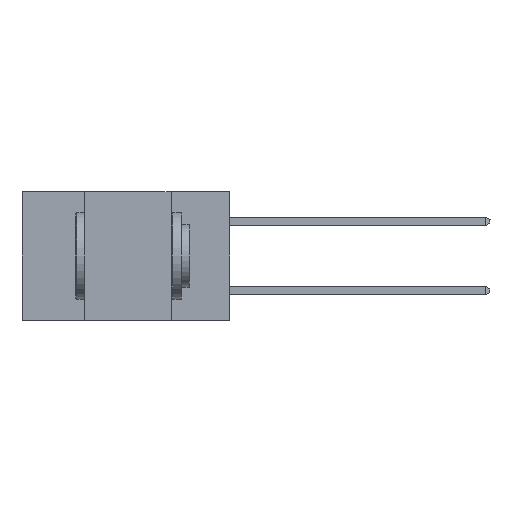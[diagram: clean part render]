
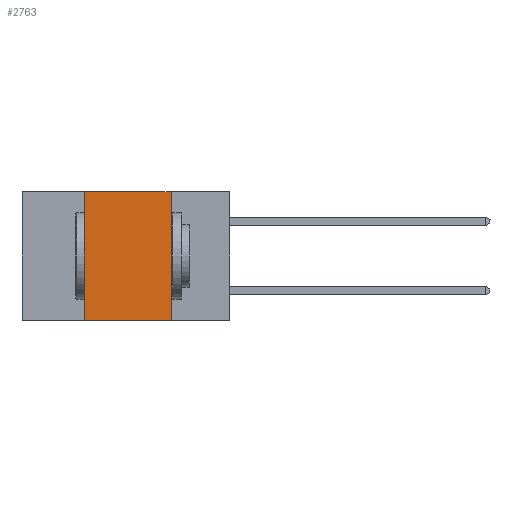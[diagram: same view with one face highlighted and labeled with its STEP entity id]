
A CAD part, left-side view. The second image highlights one B-rep face of the part: STEP entity #2763.
In plain terms, the highlighted planar face has unit normal (-1, 0, 0).
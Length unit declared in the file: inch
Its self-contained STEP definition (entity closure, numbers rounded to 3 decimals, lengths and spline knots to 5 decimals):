
#290 = VERTEX_POINT ( 'NONE', #8789 ) ;
#568 = DIRECTION ( 'NONE',  ( 1., 0., 0. ) ) ;
#764 = DIRECTION ( 'NONE',  ( 0., -1., 0. ) ) ;
#769 = VERTEX_POINT ( 'NONE', #9444 ) ;
#1569 = CARTESIAN_POINT ( 'NONE',  ( 0., 0.42, 0. ) ) ;
#1583 = DIRECTION ( 'NONE',  ( 0., -1., 0. ) ) ;
#1721 = CARTESIAN_POINT ( 'NONE',  ( 0., 0.42, -0.37 ) ) ;
#1815 = EDGE_CURVE ( 'NONE', #769, #290, #9017, .T. ) ;
#2076 = ORIENTED_EDGE ( 'NONE', *, *, #7201, .F. ) ;
#2254 = VECTOR ( 'NONE', #1583, 39.37008 ) ;
#2491 = EDGE_CURVE ( 'NONE', #769, #8243, #9269, .T. ) ;
#2763 = ADVANCED_FACE ( 'NONE', ( #6530 ), #3985, .F. ) ;
#3985 = PLANE ( 'NONE',  #6488 ) ;
#4505 = EDGE_LOOP ( 'NONE', ( #5559, #2076, #7973, #5014 ) ) ;
#5014 = ORIENTED_EDGE ( 'NONE', *, *, #1815, .T. ) ;
#5404 = DIRECTION ( 'NONE',  ( 0., 0., -1. ) ) ;
#5559 = ORIENTED_EDGE ( 'NONE', *, *, #7549, .F. ) ;
#5630 = DIRECTION ( 'NONE',  ( 0., 0., -1. ) ) ;
#5981 = DIRECTION ( 'NONE',  ( 0., 0., 1. ) ) ;
#6488 = AXIS2_PLACEMENT_3D ( 'NONE', #9919, #568, #5630 ) ;
#6530 = FACE_OUTER_BOUND ( 'NONE', #4505, .T. ) ;
#7177 = LINE ( 'NONE', #10636, #7190 ) ;
#7190 = VECTOR ( 'NONE', #5404, 39.37008 ) ;
#7201 = EDGE_CURVE ( 'NONE', #8243, #8218, #10765, .T. ) ;
#7549 = EDGE_CURVE ( 'NONE', #8218, #290, #7177, .T. ) ;
#7973 = ORIENTED_EDGE ( 'NONE', *, *, #2491, .F. ) ;
#8185 = CARTESIAN_POINT ( 'NONE',  ( 0., 0.17, 0. ) ) ;
#8218 = VERTEX_POINT ( 'NONE', #8185 ) ;
#8243 = VERTEX_POINT ( 'NONE', #1569 ) ;
#8356 = CARTESIAN_POINT ( 'NONE',  ( 0., 0.6, -0.37 ) ) ;
#8393 = VECTOR ( 'NONE', #5981, 39.37008 ) ;
#8789 = CARTESIAN_POINT ( 'NONE',  ( 0., 0.17, -0.37 ) ) ;
#9017 = LINE ( 'NONE', #8356, #10222 ) ;
#9269 = LINE ( 'NONE', #1721, #8393 ) ;
#9444 = CARTESIAN_POINT ( 'NONE',  ( 0., 0.42, -0.37 ) ) ;
#9919 = CARTESIAN_POINT ( 'NONE',  ( 0., 0.6, 0. ) ) ;
#10222 = VECTOR ( 'NONE', #764, 39.37008 ) ;
#10636 = CARTESIAN_POINT ( 'NONE',  ( 0., 0.17, -0.37 ) ) ;
#10765 = LINE ( 'NONE', #10866, #2254 ) ;
#10866 = CARTESIAN_POINT ( 'NONE',  ( 0., 0.6, 0. ) ) ;
